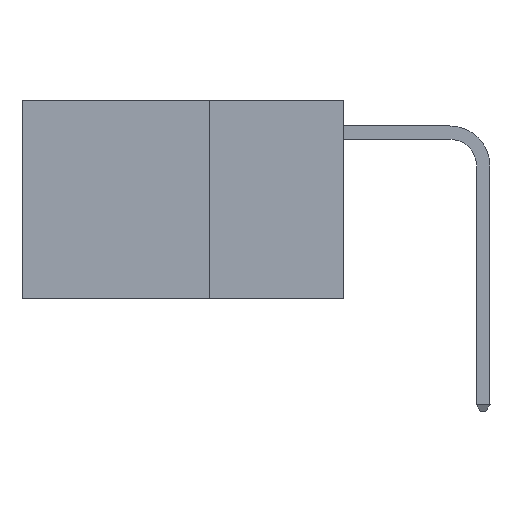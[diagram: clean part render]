
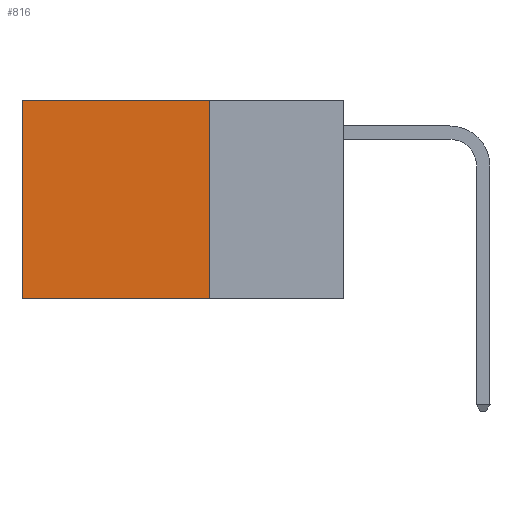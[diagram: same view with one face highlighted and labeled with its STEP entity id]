
A CAD part, left-side view. The second image highlights one B-rep face of the part: STEP entity #816.
In plain terms, the highlighted planar face has unit normal (-1, 0, 0).
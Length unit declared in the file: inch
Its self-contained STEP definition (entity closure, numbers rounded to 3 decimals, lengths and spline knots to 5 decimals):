
#816 = ADVANCED_FACE ( 'NONE', ( #7507 ), #16611, .F. ) ;
#1624 = DIRECTION ( 'NONE',  ( 0., 1., 0. ) ) ;
#1787 = DIRECTION ( 'NONE',  ( 0., 1., 0. ) ) ;
#1988 = EDGE_CURVE ( 'NONE', #27103, #16885, #13113, .T. ) ;
#2551 = AXIS2_PLACEMENT_3D ( 'NONE', #25696, #5276, #23483 ) ;
#2816 = EDGE_CURVE ( 'NONE', #10820, #27103, #8535, .T. ) ;
#2912 = ORIENTED_EDGE ( 'NONE', *, *, #1988, .F. ) ;
#2919 = VECTOR ( 'NONE', #1624, 39.37008 ) ;
#5276 = DIRECTION ( 'NONE',  ( 1., 0., 0. ) ) ;
#5315 = EDGE_CURVE ( 'NONE', #13071, #16885, #18929, .T. ) ;
#6287 = CARTESIAN_POINT ( 'NONE',  ( 0.2625, 0.25, 0. ) ) ;
#6292 = ORIENTED_EDGE ( 'NONE', *, *, #2816, .F. ) ;
#7507 = FACE_OUTER_BOUND ( 'NONE', #27457, .T. ) ;
#7734 = CARTESIAN_POINT ( 'NONE',  ( 0.2625, 0.6, 0. ) ) ;
#8353 = CARTESIAN_POINT ( 'NONE',  ( 0.2625, 0.25, -0.37 ) ) ;
#8535 = LINE ( 'NONE', #24658, #29166 ) ;
#8545 = CARTESIAN_POINT ( 'NONE',  ( 0.2625, 0.25, 0. ) ) ;
#8687 = CARTESIAN_POINT ( 'NONE',  ( 0.2625, 0.6, -0.37 ) ) ;
#10776 = DIRECTION ( 'NONE',  ( 0., 0., -1. ) ) ;
#10820 = VERTEX_POINT ( 'NONE', #8545 ) ;
#11596 = ORIENTED_EDGE ( 'NONE', *, *, #5315, .T. ) ;
#11910 = CARTESIAN_POINT ( 'NONE',  ( 0.2625, 0.6, 0. ) ) ;
#11912 = ORIENTED_EDGE ( 'NONE', *, *, #12473, .T. ) ;
#12473 = EDGE_CURVE ( 'NONE', #10820, #13071, #22398, .T. ) ;
#13071 = VERTEX_POINT ( 'NONE', #11910 ) ;
#13113 = LINE ( 'NONE', #8353, #2919 ) ;
#16611 = PLANE ( 'NONE',  #2551 ) ;
#16885 = VERTEX_POINT ( 'NONE', #8687 ) ;
#18929 = LINE ( 'NONE', #7734, #26253 ) ;
#20874 = VECTOR ( 'NONE', #1787, 39.37008 ) ;
#22398 = LINE ( 'NONE', #6287, #20874 ) ;
#23483 = DIRECTION ( 'NONE',  ( 0., 0., -1. ) ) ;
#24658 = CARTESIAN_POINT ( 'NONE',  ( 0.2625, 0.25, 0. ) ) ;
#25696 = CARTESIAN_POINT ( 'NONE',  ( 0.2625, 0.25, 0. ) ) ;
#26253 = VECTOR ( 'NONE', #28000, 39.37008 ) ;
#27103 = VERTEX_POINT ( 'NONE', #28019 ) ;
#27457 = EDGE_LOOP ( 'NONE', ( #11596, #2912, #6292, #11912 ) ) ;
#28000 = DIRECTION ( 'NONE',  ( 0., 0., -1. ) ) ;
#28019 = CARTESIAN_POINT ( 'NONE',  ( 0.2625, 0.25, -0.37 ) ) ;
#29166 = VECTOR ( 'NONE', #10776, 39.37008 ) ;
